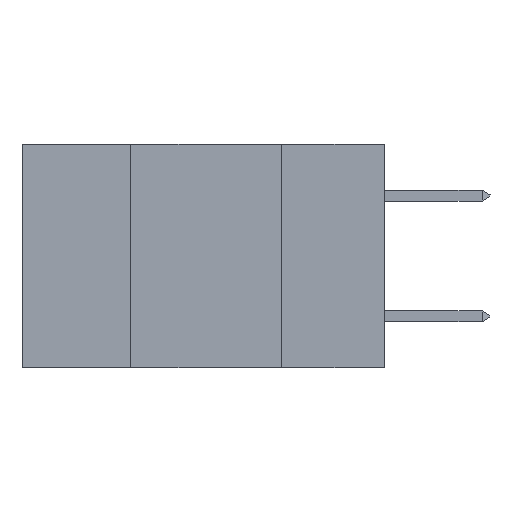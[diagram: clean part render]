
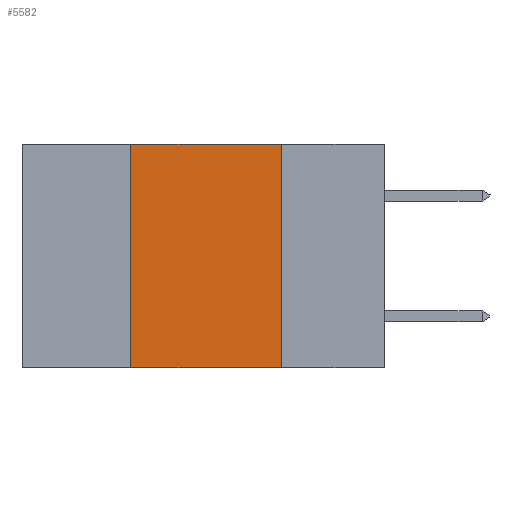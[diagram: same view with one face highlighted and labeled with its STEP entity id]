
A CAD part, left-side view. The second image highlights one B-rep face of the part: STEP entity #5582.
In plain terms, the highlighted planar face has unit normal (-1, 0, 0).
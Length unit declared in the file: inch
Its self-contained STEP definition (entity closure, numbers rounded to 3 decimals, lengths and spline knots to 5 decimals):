
#313 = VECTOR ( 'NONE', #5269, 39.37008 ) ;
#876 = PLANE ( 'NONE',  #9636 ) ;
#1336 = CARTESIAN_POINT ( 'NONE',  ( 0., 0.17, -0.37 ) ) ;
#1586 = EDGE_CURVE ( 'NONE', #11147, #13216, #14641, .T. ) ;
#1779 = LINE ( 'NONE', #4361, #6102 ) ;
#3371 = DIRECTION ( 'NONE',  ( 0., 0., -1. ) ) ;
#3394 = EDGE_CURVE ( 'NONE', #11147, #8434, #1779, .T. ) ;
#3468 = VECTOR ( 'NONE', #12852, 39.37008 ) ;
#4361 = CARTESIAN_POINT ( 'NONE',  ( 0., 0.6, -0.37 ) ) ;
#5201 = LINE ( 'NONE', #6219, #14827 ) ;
#5269 = DIRECTION ( 'NONE',  ( 0., 0., 1. ) ) ;
#5438 = FACE_OUTER_BOUND ( 'NONE', #10280, .T. ) ;
#5582 = ADVANCED_FACE ( 'NONE', ( #5438 ), #876, .F. ) ;
#6048 = VERTEX_POINT ( 'NONE', #16010 ) ;
#6102 = VECTOR ( 'NONE', #12520, 39.37008 ) ;
#6168 = CARTESIAN_POINT ( 'NONE',  ( 0., 0.17, 0. ) ) ;
#6219 = CARTESIAN_POINT ( 'NONE',  ( 0., 0.6, 0. ) ) ;
#7236 = CARTESIAN_POINT ( 'NONE',  ( 0., 0.42, 0. ) ) ;
#8396 = ORIENTED_EDGE ( 'NONE', *, *, #16617, .F. ) ;
#8434 = VERTEX_POINT ( 'NONE', #1336 ) ;
#8445 = ORIENTED_EDGE ( 'NONE', *, *, #3394, .T. ) ;
#8927 = DIRECTION ( 'NONE',  ( 0., -1., 0. ) ) ;
#9636 = AXIS2_PLACEMENT_3D ( 'NONE', #16419, #13982, #3371 ) ;
#10280 = EDGE_LOOP ( 'NONE', ( #15179, #8396, #11037, #8445 ) ) ;
#11037 = ORIENTED_EDGE ( 'NONE', *, *, #1586, .F. ) ;
#11147 = VERTEX_POINT ( 'NONE', #15519 ) ;
#12520 = DIRECTION ( 'NONE',  ( 0., -1., 0. ) ) ;
#12852 = DIRECTION ( 'NONE',  ( 0., 0., -1. ) ) ;
#13163 = CARTESIAN_POINT ( 'NONE',  ( 0., 0.42, 0. ) ) ;
#13216 = VERTEX_POINT ( 'NONE', #7236 ) ;
#13982 = DIRECTION ( 'NONE',  ( 1., 0., 0. ) ) ;
#14641 = LINE ( 'NONE', #13163, #313 ) ;
#14827 = VECTOR ( 'NONE', #8927, 39.37008 ) ;
#15068 = EDGE_CURVE ( 'NONE', #6048, #8434, #15974, .T. ) ;
#15179 = ORIENTED_EDGE ( 'NONE', *, *, #15068, .F. ) ;
#15519 = CARTESIAN_POINT ( 'NONE',  ( 0., 0.42, -0.37 ) ) ;
#15974 = LINE ( 'NONE', #6168, #3468 ) ;
#16010 = CARTESIAN_POINT ( 'NONE',  ( 0., 0.17, 0. ) ) ;
#16419 = CARTESIAN_POINT ( 'NONE',  ( 0., 0.6, 0. ) ) ;
#16617 = EDGE_CURVE ( 'NONE', #13216, #6048, #5201, .T. ) ;
